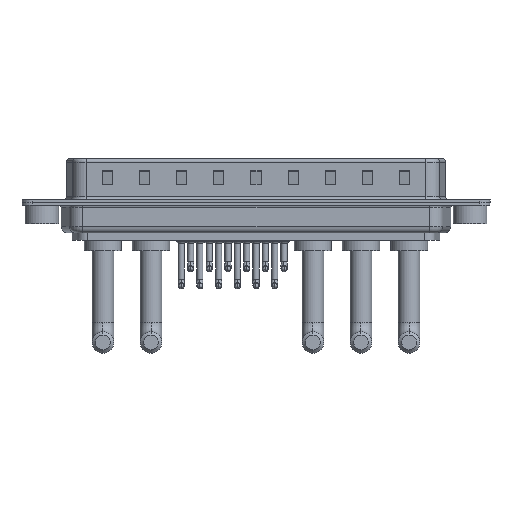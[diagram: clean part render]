
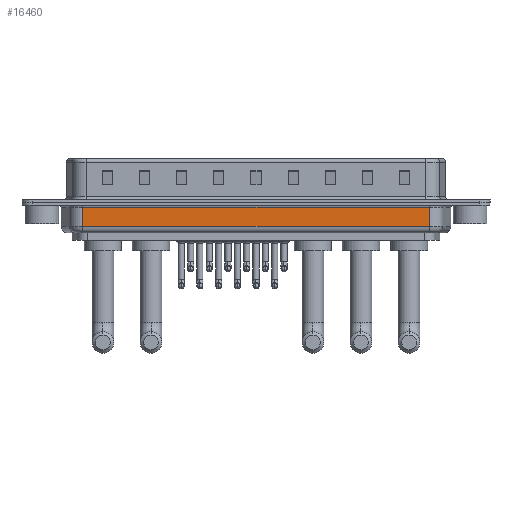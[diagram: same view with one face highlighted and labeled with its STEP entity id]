
A CAD part, front view. The second image highlights one B-rep face of the part: STEP entity #16460.
In plain terms, the highlighted planar face has unit normal (0, -1, 0).
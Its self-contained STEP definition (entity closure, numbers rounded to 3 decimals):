
#84 = CARTESIAN_POINT ( 'NONE',  ( 6.031, -5.35, -0.65 ) ) ;
#2026 = VERTEX_POINT ( 'NONE', #8415 ) ;
#3064 = LINE ( 'NONE', #24864, #4382 ) ;
#3743 = DIRECTION ( 'NONE',  ( -1., 0., 0. ) ) ;
#4382 = VECTOR ( 'NONE', #20576, 1000. ) ;
#4771 = DIRECTION ( 'NONE',  ( 0., 0., 1. ) ) ;
#5355 = LINE ( 'NONE', #7297, #14854 ) ;
#5356 = VECTOR ( 'NONE', #4771, 1000. ) ;
#6829 = LINE ( 'NONE', #22269, #20640 ) ;
#7297 = CARTESIAN_POINT ( 'NONE',  ( 6.031, -5.35, -3.5 ) ) ;
#7424 = EDGE_LOOP ( 'NONE', ( #24804, #11542, #8280, #12956 ) ) ;
#7815 = DIRECTION ( 'NONE',  ( 1., 0., 0. ) ) ;
#8280 = ORIENTED_EDGE ( 'NONE', *, *, #21187, .T. ) ;
#8415 = CARTESIAN_POINT ( 'NONE',  ( 57.469, -5.35, -0.65 ) ) ;
#9832 = DIRECTION ( 'NONE',  ( 0., 1., 0. ) ) ;
#10874 = CARTESIAN_POINT ( 'NONE',  ( 57.469, -5.35, -3.5 ) ) ;
#11401 = PLANE ( 'NONE',  #25485 ) ;
#11542 = ORIENTED_EDGE ( 'NONE', *, *, #20474, .T. ) ;
#12447 = LINE ( 'NONE', #24222, #5356 ) ;
#12956 = ORIENTED_EDGE ( 'NONE', *, *, #23810, .T. ) ;
#12983 = CARTESIAN_POINT ( 'NONE',  ( 6.031, -5.35, -3.5 ) ) ;
#13908 = VERTEX_POINT ( 'NONE', #10874 ) ;
#14854 = VECTOR ( 'NONE', #7815, 1000. ) ;
#15337 = VERTEX_POINT ( 'NONE', #12983 ) ;
#16460 = ADVANCED_FACE ( 'NONE', ( #23332 ), #11401, .F. ) ;
#16561 = DIRECTION ( 'NONE',  ( -1., 0., 0. ) ) ;
#16731 = EDGE_CURVE ( 'NONE', #15337, #18703, #3064, .T. ) ;
#18703 = VERTEX_POINT ( 'NONE', #84 ) ;
#20474 = EDGE_CURVE ( 'NONE', #15337, #13908, #5355, .T. ) ;
#20576 = DIRECTION ( 'NONE',  ( 0., 0., 1. ) ) ;
#20640 = VECTOR ( 'NONE', #16561, 1000. ) ;
#21187 = EDGE_CURVE ( 'NONE', #13908, #2026, #12447, .T. ) ;
#22269 = CARTESIAN_POINT ( 'NONE',  ( 6.031, -5.35, -0.65 ) ) ;
#23332 = FACE_OUTER_BOUND ( 'NONE', #7424, .T. ) ;
#23810 = EDGE_CURVE ( 'NONE', #2026, #18703, #6829, .T. ) ;
#24222 = CARTESIAN_POINT ( 'NONE',  ( 57.469, -5.35, -4.5 ) ) ;
#24804 = ORIENTED_EDGE ( 'NONE', *, *, #16731, .F. ) ;
#24864 = CARTESIAN_POINT ( 'NONE',  ( 6.031, -5.35, -4.5 ) ) ;
#25399 = CARTESIAN_POINT ( 'NONE',  ( 6.031, -5.35, -4.5 ) ) ;
#25485 = AXIS2_PLACEMENT_3D ( 'NONE', #25399, #9832, #3743 ) ;
